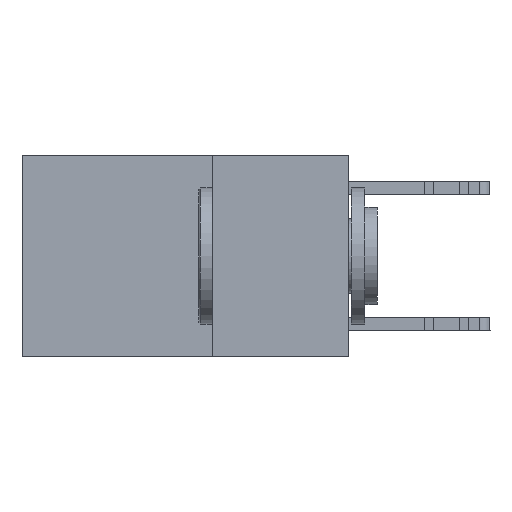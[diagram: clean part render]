
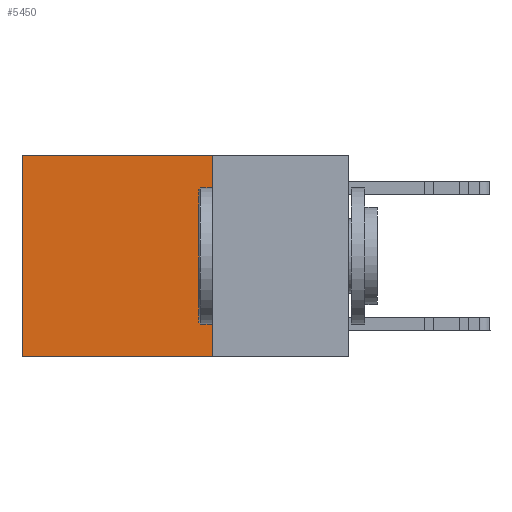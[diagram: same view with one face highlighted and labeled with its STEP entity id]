
A CAD part, left-side view. The second image highlights one B-rep face of the part: STEP entity #5450.
In plain terms, the highlighted planar face has unit normal (-1, 0, 0).
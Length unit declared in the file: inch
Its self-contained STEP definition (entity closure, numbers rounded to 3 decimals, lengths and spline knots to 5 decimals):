
#1266 = ORIENTED_EDGE ( 'NONE', *, *, #6094, .T. ) ;
#2510 = LINE ( 'NONE', #4656, #2722 ) ;
#2722 = VECTOR ( 'NONE', #12255, 39.37008 ) ;
#2917 = EDGE_CURVE ( 'NONE', #3973, #19822, #8975, .T. ) ;
#3973 = VERTEX_POINT ( 'NONE', #23355 ) ;
#4656 = CARTESIAN_POINT ( 'NONE',  ( 0.2625, 0.6, 0. ) ) ;
#4933 = VERTEX_POINT ( 'NONE', #26083 ) ;
#4988 = CARTESIAN_POINT ( 'NONE',  ( 0.2625, 0.25, -0.37 ) ) ;
#5235 = ORIENTED_EDGE ( 'NONE', *, *, #8716, .F. ) ;
#5436 = EDGE_LOOP ( 'NONE', ( #1266, #15778, #5235, #31658 ) ) ;
#5450 = ADVANCED_FACE ( 'NONE', ( #19230 ), #11975, .F. ) ;
#6094 = EDGE_CURVE ( 'NONE', #19822, #4933, #2510, .T. ) ;
#6502 = DIRECTION ( 'NONE',  ( 0., 1., 0. ) ) ;
#6931 = DIRECTION ( 'NONE',  ( 0., 1., 0. ) ) ;
#8519 = VECTOR ( 'NONE', #22528, 39.37008 ) ;
#8716 = EDGE_CURVE ( 'NONE', #3973, #9173, #32086, .T. ) ;
#8975 = LINE ( 'NONE', #19047, #10955 ) ;
#9173 = VERTEX_POINT ( 'NONE', #4988 ) ;
#9489 = VECTOR ( 'NONE', #6931, 39.37008 ) ;
#9605 = EDGE_CURVE ( 'NONE', #9173, #4933, #24936, .T. ) ;
#10955 = VECTOR ( 'NONE', #6502, 39.37008 ) ;
#11975 = PLANE ( 'NONE',  #23858 ) ;
#12255 = DIRECTION ( 'NONE',  ( 0., 0., -1. ) ) ;
#15778 = ORIENTED_EDGE ( 'NONE', *, *, #9605, .F. ) ;
#19047 = CARTESIAN_POINT ( 'NONE',  ( 0.2625, 0.25, 0. ) ) ;
#19230 = FACE_OUTER_BOUND ( 'NONE', #5436, .T. ) ;
#19822 = VERTEX_POINT ( 'NONE', #26944 ) ;
#22528 = DIRECTION ( 'NONE',  ( 0., 0., -1. ) ) ;
#23355 = CARTESIAN_POINT ( 'NONE',  ( 0.2625, 0.25, 0. ) ) ;
#23858 = AXIS2_PLACEMENT_3D ( 'NONE', #29307, #26651, #32085 ) ;
#24769 = CARTESIAN_POINT ( 'NONE',  ( 0.2625, 0.25, -0.37 ) ) ;
#24936 = LINE ( 'NONE', #24769, #9489 ) ;
#26083 = CARTESIAN_POINT ( 'NONE',  ( 0.2625, 0.6, -0.37 ) ) ;
#26651 = DIRECTION ( 'NONE',  ( 1., 0., 0. ) ) ;
#26944 = CARTESIAN_POINT ( 'NONE',  ( 0.2625, 0.6, 0. ) ) ;
#29307 = CARTESIAN_POINT ( 'NONE',  ( 0.2625, 0.25, 0. ) ) ;
#29637 = CARTESIAN_POINT ( 'NONE',  ( 0.2625, 0.25, 0. ) ) ;
#31658 = ORIENTED_EDGE ( 'NONE', *, *, #2917, .T. ) ;
#32085 = DIRECTION ( 'NONE',  ( 0., 0., -1. ) ) ;
#32086 = LINE ( 'NONE', #29637, #8519 ) ;
